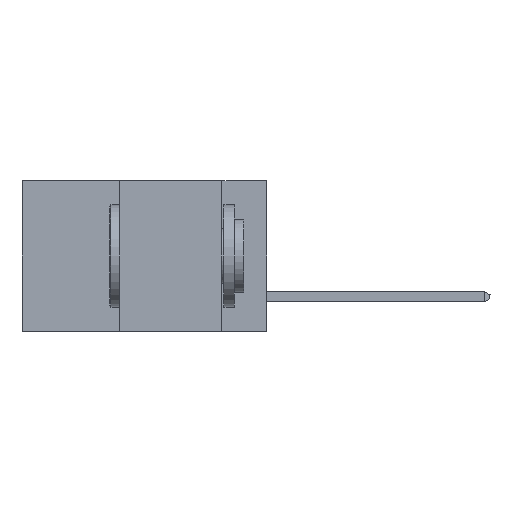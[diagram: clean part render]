
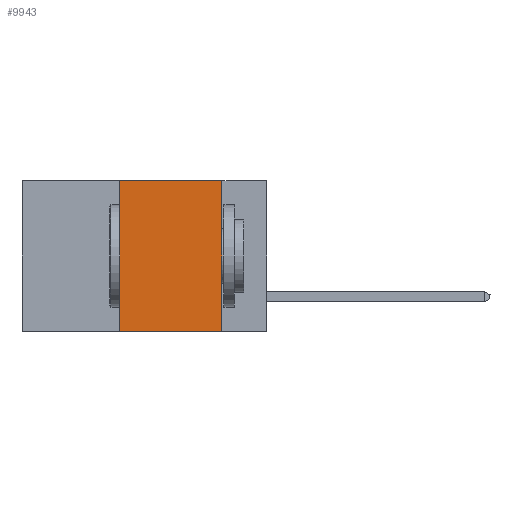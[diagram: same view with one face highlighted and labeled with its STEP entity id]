
A CAD part, left-side view. The second image highlights one B-rep face of the part: STEP entity #9943.
In plain terms, the highlighted planar face has unit normal (-1, 0, 0).
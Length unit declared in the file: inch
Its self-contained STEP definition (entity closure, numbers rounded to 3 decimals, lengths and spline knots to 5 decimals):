
#1566 = CARTESIAN_POINT ( 'NONE',  ( 0., 0.11, -0.37 ) ) ;
#1639 = LINE ( 'NONE', #36252, #45509 ) ;
#1776 = VERTEX_POINT ( 'NONE', #39325 ) ;
#2228 = DIRECTION ( 'NONE',  ( 1., 0., 0. ) ) ;
#2487 = ORIENTED_EDGE ( 'NONE', *, *, #26267, .T. ) ;
#2749 = EDGE_CURVE ( 'NONE', #26384, #12887, #15537, .T. ) ;
#3682 = LINE ( 'NONE', #20630, #4812 ) ;
#4812 = VECTOR ( 'NONE', #7125, 39.37008 ) ;
#6473 = ORIENTED_EDGE ( 'NONE', *, *, #15090, .F. ) ;
#6520 = EDGE_LOOP ( 'NONE', ( #36050, #6473, #44651, #2487 ) ) ;
#7125 = DIRECTION ( 'NONE',  ( 0., -1., 0. ) ) ;
#9917 = VERTEX_POINT ( 'NONE', #1566 ) ;
#9943 = ADVANCED_FACE ( 'NONE', ( #11187 ), #20317, .F. ) ;
#11166 = DIRECTION ( 'NONE',  ( 0., 0., -1. ) ) ;
#11187 = FACE_OUTER_BOUND ( 'NONE', #6520, .T. ) ;
#12887 = VERTEX_POINT ( 'NONE', #28740 ) ;
#14506 = DIRECTION ( 'NONE',  ( 0., -1., 0. ) ) ;
#15090 = EDGE_CURVE ( 'NONE', #12887, #1776, #3682, .T. ) ;
#15537 = LINE ( 'NONE', #15655, #24658 ) ;
#15655 = CARTESIAN_POINT ( 'NONE',  ( 0., 0.36, 0. ) ) ;
#19868 = LINE ( 'NONE', #26117, #22679 ) ;
#20317 = PLANE ( 'NONE',  #25630 ) ;
#20630 = CARTESIAN_POINT ( 'NONE',  ( 0., 0.6, 0. ) ) ;
#22679 = VECTOR ( 'NONE', #11166, 39.37008 ) ;
#23988 = EDGE_CURVE ( 'NONE', #1776, #9917, #19868, .T. ) ;
#24658 = VECTOR ( 'NONE', #44301, 39.37008 ) ;
#25630 = AXIS2_PLACEMENT_3D ( 'NONE', #41880, #2228, #31060 ) ;
#26117 = CARTESIAN_POINT ( 'NONE',  ( 0., 0.11, 0. ) ) ;
#26267 = EDGE_CURVE ( 'NONE', #26384, #9917, #1639, .T. ) ;
#26384 = VERTEX_POINT ( 'NONE', #37022 ) ;
#28740 = CARTESIAN_POINT ( 'NONE',  ( 0., 0.36, 0. ) ) ;
#31060 = DIRECTION ( 'NONE',  ( 0., 0., -1. ) ) ;
#36050 = ORIENTED_EDGE ( 'NONE', *, *, #23988, .F. ) ;
#36252 = CARTESIAN_POINT ( 'NONE',  ( 0., 0.6, -0.37 ) ) ;
#37022 = CARTESIAN_POINT ( 'NONE',  ( 0., 0.36, -0.37 ) ) ;
#39325 = CARTESIAN_POINT ( 'NONE',  ( 0., 0.11, 0. ) ) ;
#41880 = CARTESIAN_POINT ( 'NONE',  ( 0., 0.6, 0. ) ) ;
#44301 = DIRECTION ( 'NONE',  ( 0., 0., 1. ) ) ;
#44651 = ORIENTED_EDGE ( 'NONE', *, *, #2749, .F. ) ;
#45509 = VECTOR ( 'NONE', #14506, 39.37008 ) ;
